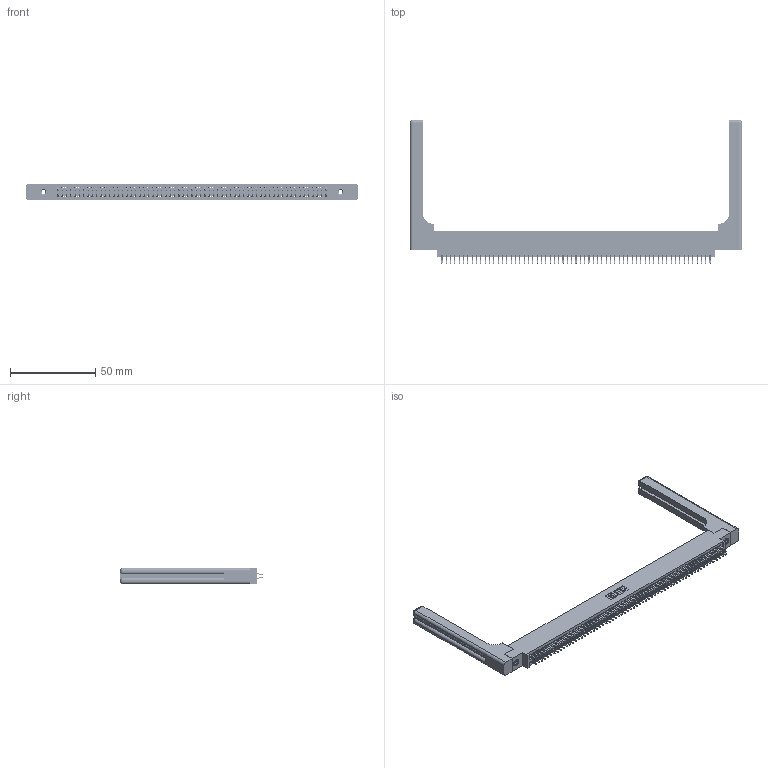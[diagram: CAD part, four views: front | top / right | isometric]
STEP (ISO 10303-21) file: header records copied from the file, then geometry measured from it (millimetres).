
FILE_DESCRIPTION (( 'STEP AP203' ), '1' );
FILE_NAME ('345-126-556-858.STEP', '2019-11-07T05:27:37', ( '' ), ( '' ), 'SwSTEP 2.0', 'SolidWorks 2016', '' );
FILE_SCHEMA (( 'CONFIG_CONTROL_DESIGN' ));
Length unit declared in the file: inch
Products named in the file (5): 345-292-001_556 Tail; 345 Part_0.170 Offset - 0.156 Dia-TH; 345-126-556-858; 345-250-001_345-250-001-102; 345-220-058_345-220-058
Assembly tree (131 placements, depth 2):
  345-126-556-858
    345 Part_0.170 Offset - 0.156 Dia-TH
    345-292-001_556 Tail  x126
    345-250-001_345-250-001-102  x2
    345-220-058_345-220-058  x2
Bounding box: 195.05 x 84.51 x 9.4 mm (x, y, z)
Volume: 27498.7 mm3; surface area: 33618.8 mm2
Topology: 131 solids, 131 shells, 7442 faces, 22061 edges, 14518 vertices
Faces by surface type: plane 4894, cylinder 2488, bspline 36, cone 12, sphere 8, torus 4
Entity records: 52138 total; most frequent: CARTESIAN_POINT 9729, ORIENTED_EDGE 8448, DIRECTION 7472, EDGE_CURVE 4224, LINE 3740, VECTOR 3740, VERTEX_POINT 2806, AXIS2_PLACEMENT_3D 1866
